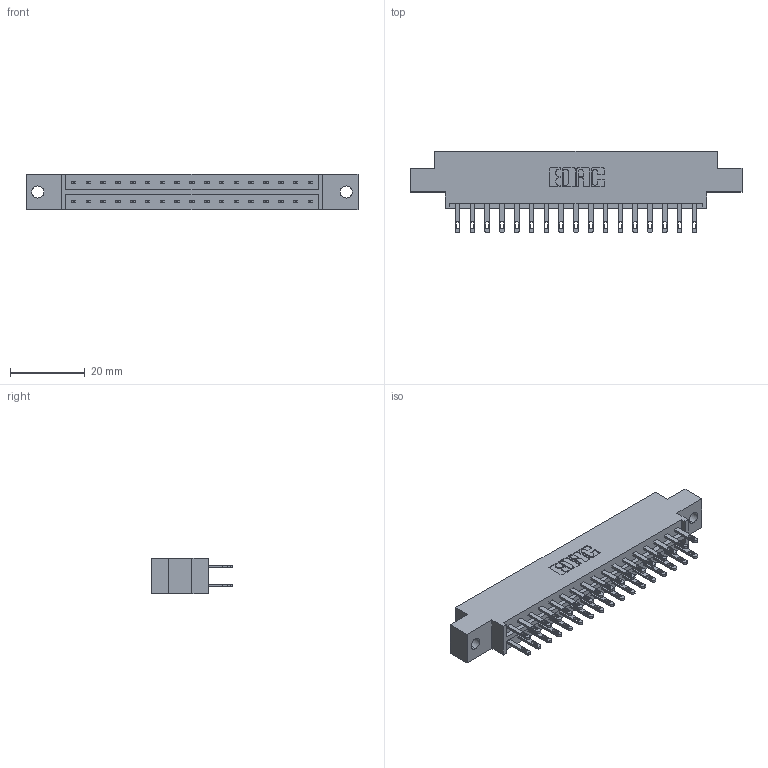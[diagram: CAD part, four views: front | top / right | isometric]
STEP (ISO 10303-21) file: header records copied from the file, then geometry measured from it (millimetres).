
FILE_DESCRIPTION (( 'STEP AP203' ), '1' );
FILE_NAME ('833-034-500-802.STEP', '2020-06-02T21:06:51', ( '' ), ( '' ), 'SwSTEP 2.0', 'SolidWorks 2020', '' );
FILE_SCHEMA (( 'CONFIG_CONTROL_DESIGN' ));
Length unit declared in the file: inch
Products named in the file (3): 345-292-001_345-293-100; 833-034-500-802; 833 Part_Offset - .128 Dia
Assembly tree (35 placements, depth 2):
  833-034-500-802
    833 Part_Offset - .128 Dia
    345-292-001_345-293-100  x34
Bounding box: 88.9 x 21.85 x 9.4 mm (x, y, z)
Volume: 8681.8 mm3; surface area: 10317.1 mm2
Topology: 35 solids, 35 shells, 1750 faces, 5321 edges, 3546 vertices
Faces by surface type: plane 1094, cylinder 656
Entity records: 14235 total; most frequent: CARTESIAN_POINT 2390, ORIENTED_EDGE 2326, DIRECTION 2087, EDGE_CURVE 1163, VECTOR 1031, LINE 1031, VERTEX_POINT 774, AXIS2_PLACEMENT_3D 528
